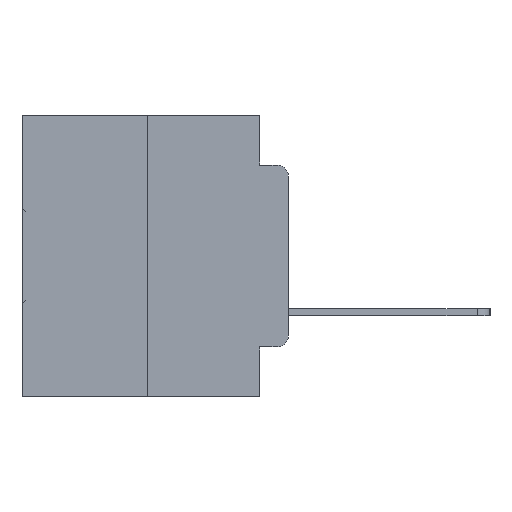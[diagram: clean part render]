
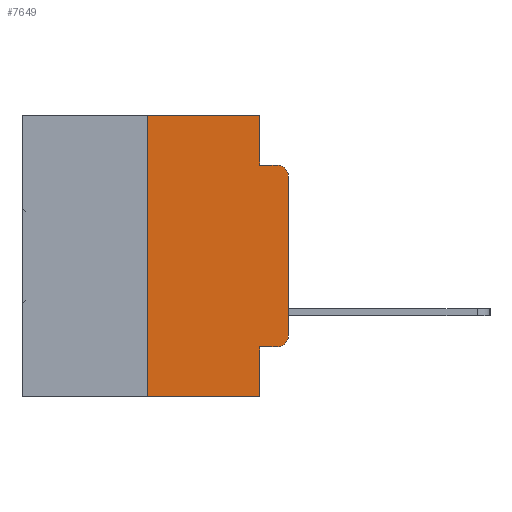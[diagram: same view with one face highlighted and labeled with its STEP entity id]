
A CAD part, left-side view. The second image highlights one B-rep face of the part: STEP entity #7649.
In plain terms, the highlighted planar face has unit normal (-1, 0, 0).
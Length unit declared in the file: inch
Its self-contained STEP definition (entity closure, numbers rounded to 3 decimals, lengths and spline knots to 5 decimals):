
#102 = LINE ( 'NONE', #1456, #12561 ) ;
#1177 = DIRECTION ( 'NONE',  ( -1., 0., 0. ) ) ;
#1456 = CARTESIAN_POINT ( 'NONE',  ( 0., 0.051, 0. ) ) ;
#1592 = EDGE_CURVE ( 'NONE', #18789, #11049, #10127, .T. ) ;
#2236 = DIRECTION ( 'NONE',  ( 0., 0., -1. ) ) ;
#2512 = CIRCLE ( 'NONE', #14139, 0.02 ) ;
#2732 = VECTOR ( 'NONE', #18498, 39.37008 ) ;
#2981 = VERTEX_POINT ( 'NONE', #16809 ) ;
#3037 = CARTESIAN_POINT ( 'NONE',  ( 0., 0.25, 0. ) ) ;
#3141 = DIRECTION ( 'NONE',  ( 0., -1., 0. ) ) ;
#3467 = VECTOR ( 'NONE', #3922, 39.37008 ) ;
#3922 = DIRECTION ( 'NONE',  ( 0., -1., 0. ) ) ;
#4200 = ORIENTED_EDGE ( 'NONE', *, *, #29725, .T. ) ;
#5042 = DIRECTION ( 'NONE',  ( -1., 0., 0. ) ) ;
#6250 = CARTESIAN_POINT ( 'NONE',  ( 0., 0.051, 0. ) ) ;
#6303 = CARTESIAN_POINT ( 'NONE',  ( 0., 0.051, -0.0885 ) ) ;
#6405 = CARTESIAN_POINT ( 'NONE',  ( 0., 0.051, -0.0885 ) ) ;
#6552 = CARTESIAN_POINT ( 'NONE',  ( 0., 0.02, -0.4115 ) ) ;
#7649 = ADVANCED_FACE ( 'NONE', ( #30240 ), #14578, .F. ) ;
#7876 = EDGE_CURVE ( 'NONE', #18731, #12172, #11236, .T. ) ;
#8482 = LINE ( 'NONE', #30246, #20718 ) ;
#8704 = VERTEX_POINT ( 'NONE', #6552 ) ;
#8756 = CARTESIAN_POINT ( 'NONE',  ( 0., 0., 0. ) ) ;
#9641 = CARTESIAN_POINT ( 'NONE',  ( 0., 0.473, 0. ) ) ;
#10127 = LINE ( 'NONE', #6250, #2732 ) ;
#11049 = VERTEX_POINT ( 'NONE', #23054 ) ;
#11236 = LINE ( 'NONE', #17881, #23417 ) ;
#11320 = ORIENTED_EDGE ( 'NONE', *, *, #12431, .F. ) ;
#11691 = VECTOR ( 'NONE', #27346, 39.37008 ) ;
#12172 = VERTEX_POINT ( 'NONE', #3037 ) ;
#12421 = AXIS2_PLACEMENT_3D ( 'NONE', #9641, #17032, #2236 ) ;
#12431 = EDGE_CURVE ( 'NONE', #2981, #13698, #102, .T. ) ;
#12561 = VECTOR ( 'NONE', #30766, 39.37008 ) ;
#13089 = VERTEX_POINT ( 'NONE', #21016 ) ;
#13391 = EDGE_CURVE ( 'NONE', #8704, #29457, #17474, .T. ) ;
#13698 = VERTEX_POINT ( 'NONE', #6303 ) ;
#14139 = AXIS2_PLACEMENT_3D ( 'NONE', #16019, #1177, #18465 ) ;
#14540 = EDGE_LOOP ( 'NONE', ( #22215, #4200, #25305, #11320, #28965, #16589, #22948, #22970, #26326, #14820 ) ) ;
#14578 = PLANE ( 'NONE',  #12421 ) ;
#14820 = ORIENTED_EDGE ( 'NONE', *, *, #13391, .T. ) ;
#15961 = VECTOR ( 'NONE', #18606, 39.37008 ) ;
#16019 = CARTESIAN_POINT ( 'NONE',  ( 0., 0.02, -0.1085 ) ) ;
#16589 = ORIENTED_EDGE ( 'NONE', *, *, #7876, .F. ) ;
#16625 = EDGE_CURVE ( 'NONE', #12172, #2981, #31259, .T. ) ;
#16809 = CARTESIAN_POINT ( 'NONE',  ( 0., 0.051, 0. ) ) ;
#17032 = DIRECTION ( 'NONE',  ( 1., 0., 0. ) ) ;
#17474 = CIRCLE ( 'NONE', #20513, 0.02 ) ;
#17625 = VECTOR ( 'NONE', #3141, 39.37008 ) ;
#17881 = CARTESIAN_POINT ( 'NONE',  ( 0., 0.25, 0. ) ) ;
#18465 = DIRECTION ( 'NONE',  ( 0., 0., -1. ) ) ;
#18498 = DIRECTION ( 'NONE',  ( 0., 0., -1. ) ) ;
#18606 = DIRECTION ( 'NONE',  ( 0., 0., 1. ) ) ;
#18731 = VERTEX_POINT ( 'NONE', #18960 ) ;
#18789 = VERTEX_POINT ( 'NONE', #24045 ) ;
#18960 = CARTESIAN_POINT ( 'NONE',  ( 0., 0.25, -0.5 ) ) ;
#19713 = CARTESIAN_POINT ( 'NONE',  ( 0., 0.02, -0.3915 ) ) ;
#20319 = DIRECTION ( 'NONE',  ( 0., 0., 1. ) ) ;
#20513 = AXIS2_PLACEMENT_3D ( 'NONE', #19713, #5042, #22169 ) ;
#20718 = VECTOR ( 'NONE', #31467, 39.37008 ) ;
#21016 = CARTESIAN_POINT ( 'NONE',  ( 0., 0.02, -0.0885 ) ) ;
#21230 = VERTEX_POINT ( 'NONE', #30419 ) ;
#22169 = DIRECTION ( 'NONE',  ( 0., 0., -1. ) ) ;
#22215 = ORIENTED_EDGE ( 'NONE', *, *, #31156, .T. ) ;
#22948 = ORIENTED_EDGE ( 'NONE', *, *, #23261, .T. ) ;
#22970 = ORIENTED_EDGE ( 'NONE', *, *, #1592, .F. ) ;
#23054 = CARTESIAN_POINT ( 'NONE',  ( 0., 0.051, -0.5 ) ) ;
#23166 = LINE ( 'NONE', #8756, #15961 ) ;
#23261 = EDGE_CURVE ( 'NONE', #18731, #11049, #24632, .T. ) ;
#23417 = VECTOR ( 'NONE', #20319, 39.37008 ) ;
#24045 = CARTESIAN_POINT ( 'NONE',  ( 0., 0.051, -0.4115 ) ) ;
#24609 = CARTESIAN_POINT ( 'NONE',  ( 0., 0., -0.3915 ) ) ;
#24632 = LINE ( 'NONE', #24923, #11691 ) ;
#24923 = CARTESIAN_POINT ( 'NONE',  ( 0., 0.473, -0.5 ) ) ;
#25091 = CARTESIAN_POINT ( 'NONE',  ( 0., 0.473, 0. ) ) ;
#25305 = ORIENTED_EDGE ( 'NONE', *, *, #27498, .F. ) ;
#26326 = ORIENTED_EDGE ( 'NONE', *, *, #28023, .T. ) ;
#27346 = DIRECTION ( 'NONE',  ( 0., -1., 0. ) ) ;
#27498 = EDGE_CURVE ( 'NONE', #13698, #13089, #29439, .T. ) ;
#28023 = EDGE_CURVE ( 'NONE', #18789, #8704, #8482, .T. ) ;
#28965 = ORIENTED_EDGE ( 'NONE', *, *, #16625, .F. ) ;
#29439 = LINE ( 'NONE', #6405, #3467 ) ;
#29457 = VERTEX_POINT ( 'NONE', #24609 ) ;
#29725 = EDGE_CURVE ( 'NONE', #21230, #13089, #2512, .T. ) ;
#30240 = FACE_OUTER_BOUND ( 'NONE', #14540, .T. ) ;
#30246 = CARTESIAN_POINT ( 'NONE',  ( 0., 0.051, -0.4115 ) ) ;
#30419 = CARTESIAN_POINT ( 'NONE',  ( 0., 0., -0.1085 ) ) ;
#30766 = DIRECTION ( 'NONE',  ( 0., 0., -1. ) ) ;
#31156 = EDGE_CURVE ( 'NONE', #29457, #21230, #23166, .T. ) ;
#31259 = LINE ( 'NONE', #25091, #17625 ) ;
#31467 = DIRECTION ( 'NONE',  ( 0., -1., 0. ) ) ;
